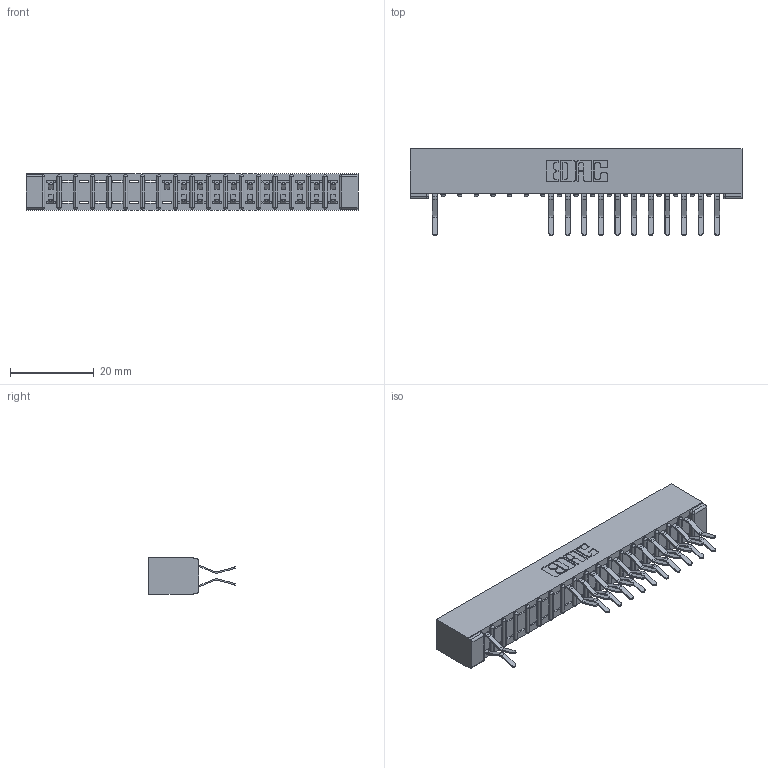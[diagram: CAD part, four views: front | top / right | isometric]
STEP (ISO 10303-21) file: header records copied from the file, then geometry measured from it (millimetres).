
FILE_DESCRIPTION (( 'STEP AP203' ), '1' );
FILE_NAME ('307-036-560-201.STEP', '2018-08-05T09:20:18', ( '' ), ( '' ), 'SwSTEP 2.0', 'SolidWorks 2016', '' );
FILE_SCHEMA (( 'CONFIG_CONTROL_DESIGN' ));
Length unit declared in the file: inch
Products named in the file (3): 307 Part_No Mounting Lugs; 307-290-001_560; 307-036-560-201
Assembly tree (24 placements, depth 2):
  307-036-560-201
    307 Part_No Mounting Lugs
    307-290-001_560  x23
Bounding box: 79.2 x 20.73 x 8.71 mm (x, y, z)
Volume: 5274.3 mm3; surface area: 8757.8 mm2
Topology: 24 solids, 24 shells, 1409 faces, 3981 edges, 2570 vertices
Faces by surface type: plane 903, cylinder 468, sphere 38
Entity records: 18376 total; most frequent: CARTESIAN_POINT 3065, ORIENTED_EDGE 3046, DIRECTION 2999, EDGE_CURVE 1523, LINE 1159, VECTOR 1159, VERTEX_POINT 986, AXIS2_PLACEMENT_3D 920
